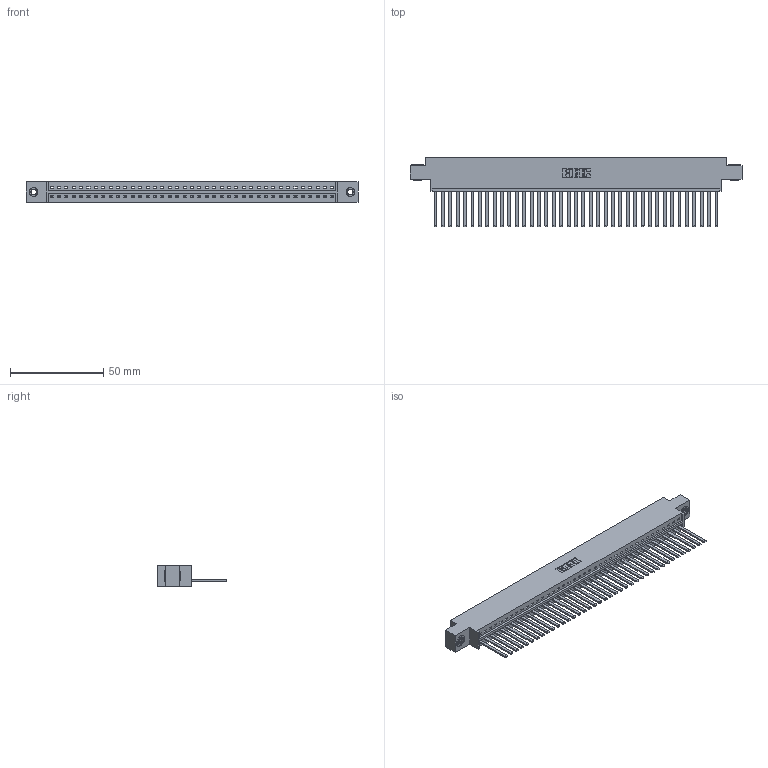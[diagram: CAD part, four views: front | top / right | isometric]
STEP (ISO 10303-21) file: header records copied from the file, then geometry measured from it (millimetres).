
FILE_DESCRIPTION (( 'STEP AP203' ), '1' );
FILE_NAME ('336-039-541-603.STEP', '2020-08-07T23:09:57', ( '' ), ( '' ), 'SwSTEP 2.0', 'SolidWorks 2020', '' );
FILE_SCHEMA (( 'CONFIG_CONTROL_DESIGN' ));
Length unit declared in the file: inch
Products named in the file (4): 345-250-002_345-250-002-102; 336 Part_Offset - .156 Dia - TH; 336-290-001_336-290-541; 336-039-541-603
Assembly tree (42 placements, depth 2):
  336-039-541-603
    336 Part_Offset - .156 Dia - TH
    336-290-001_336-290-541  x39
    345-250-002_345-250-002-102  x2
Bounding box: 177.93 x 37.34 x 11.1 mm (x, y, z)
Volume: 25856.5 mm3; surface area: 28417.1 mm2
Topology: 42 solids, 42 shells, 2106 faces, 6405 edges, 4240 vertices
Faces by surface type: plane 1410, cylinder 688, cone 8
Entity records: 29879 total; most frequent: CARTESIAN_POINT 5265, ORIENTED_EDGE 5134, DIRECTION 4375, EDGE_CURVE 2567, VECTOR 2411, LINE 2411, VERTEX_POINT 1708, AXIS2_PLACEMENT_3D 982
